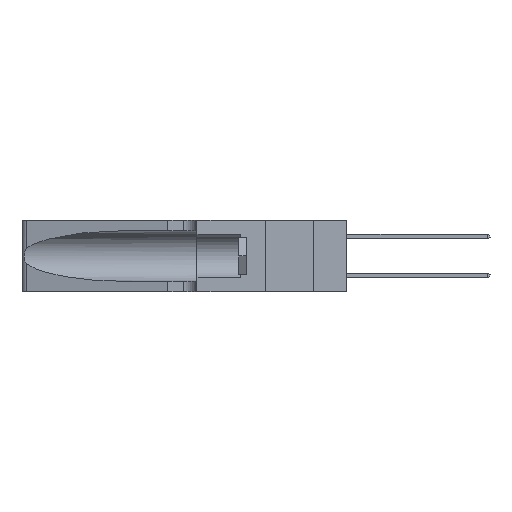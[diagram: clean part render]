
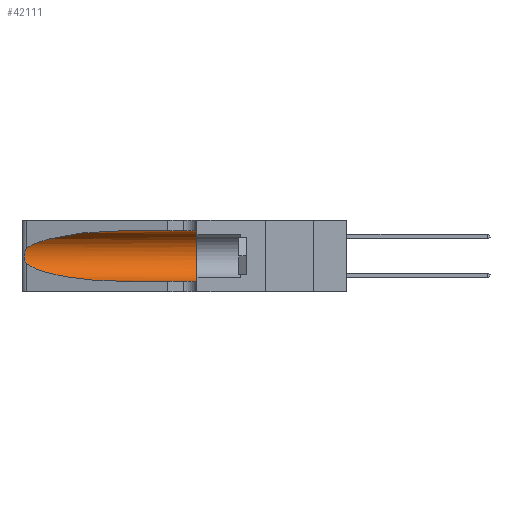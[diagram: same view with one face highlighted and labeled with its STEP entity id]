
A CAD part, left-side view. The second image highlights one B-rep face of the part: STEP entity #42111.
In plain terms, the highlighted cylindrical face has radius 3.308 mm (diameter 6.617 mm), a partial arc.
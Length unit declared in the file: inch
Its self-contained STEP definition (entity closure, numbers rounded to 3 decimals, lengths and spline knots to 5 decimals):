
#189 = DIRECTION ( 'NONE',  ( 0., -1., 0. ) ) ;
#308 = LINE ( 'NONE', #18726, #39827 ) ;
#416 = EDGE_CURVE ( 'NONE', #18022, #40459, #35039, .T. ) ;
#1142 = FACE_OUTER_BOUND ( 'NONE', #48727, .T. ) ;
#2144 = LINE ( 'NONE', #30897, #41596 ) ;
#3174 = CARTESIAN_POINT ( 'NONE',  ( 0.26075, 1.23896, 0.19203 ) ) ;
#3382 = DIRECTION ( 'NONE',  ( 0., 0., 1. ) ) ;
#7046 = CARTESIAN_POINT ( 'NONE',  ( 0.26017, 1.23833, 0.17102 ) ) ;
#7068 = VERTEX_POINT ( 'NONE', #26553 ) ;
#7631 = EDGE_CURVE ( 'NONE', #7068, #35175, #38457, .T. ) ;
#7908 = EDGE_CURVE ( 'NONE', #14435, #7068, #29641, .T. ) ;
#8144 =( BOUNDED_CURVE ( )  B_SPLINE_CURVE ( 3, ( #31786, #16528, #46935, #24254 ),
 .UNSPECIFIED., .F., .F. ) 
 B_SPLINE_CURVE_WITH_KNOTS ( ( 4, 4 ),
 ( 3.44316, 4.71239 ),
 .UNSPECIFIED. ) 
 CURVE ( )  GEOMETRIC_REPRESENTATION_ITEM ( )  RATIONAL_B_SPLINE_CURVE ( ( 1., 0.87, 0.87, 1. ) ) 
 REPRESENTATION_ITEM ( '' )  );
#10740 = CARTESIAN_POINT ( 'NONE',  ( 0.25555, 1.22994, 0.2215 ) ) ;
#10910 = CARTESIAN_POINT ( 'NONE',  ( 0.25789, 1.23486, 0.15765 ) ) ;
#12070 = ORIENTED_EDGE ( 'NONE', *, *, #41058, .T. ) ;
#12370 = CARTESIAN_POINT ( 'NONE',  ( 0.2373, 1.15595, 0.28018 ) ) ;
#14435 = VERTEX_POINT ( 'NONE', #36210 ) ;
#14732 = CARTESIAN_POINT ( 'NONE',  ( 0.25555, 1.22993, 0.14849 ) ) ;
#15264 = ORIENTED_EDGE ( 'NONE', *, *, #7908, .T. ) ;
#16361 = AXIS2_PLACEMENT_3D ( 'NONE', #46184, #19645, #23495 ) ;
#16528 = CARTESIAN_POINT ( 'NONE',  ( 0.2373, 1.15595, 0.08982 ) ) ;
#16903 = ORIENTED_EDGE ( 'NONE', *, *, #416, .F. ) ;
#17095 = ORIENTED_EDGE ( 'NONE', *, *, #7631, .T. ) ;
#18022 = VERTEX_POINT ( 'NONE', #38744 ) ;
#18726 = CARTESIAN_POINT ( 'NONE',  ( 0.1305, 1.61858, 0.31525 ) ) ;
#19645 = DIRECTION ( 'NONE',  ( 0., -1., 0. ) ) ;
#21640 = CARTESIAN_POINT ( 'NONE',  ( 0.25487, 1.22718, 0.14631 ) ) ;
#22294 = CARTESIAN_POINT ( 'NONE',  ( 0.25787, 1.23484, 0.2124 ) ) ;
#23495 = DIRECTION ( 'NONE',  ( 0., 0., -1. ) ) ;
#24254 = CARTESIAN_POINT ( 'NONE',  ( 0.1305, 0.72297, 0.05475 ) ) ;
#25541 = VERTEX_POINT ( 'NONE', #34522 ) ;
#26155 = CARTESIAN_POINT ( 'NONE',  ( 0.26018, 1.23835, 0.19895 ) ) ;
#26376 = DIRECTION ( 'NONE',  ( 0., 1., 0. ) ) ;
#26553 = CARTESIAN_POINT ( 'NONE',  ( 0.25487, 1.22718, 0.22369 ) ) ;
#27500 = EDGE_CURVE ( 'NONE', #25541, #40459, #2144, .T. ) ;
#29641 =( BOUNDED_CURVE ( )  B_SPLINE_CURVE ( 3, ( #31464, #35264, #12370, #39073 ),
 .UNSPECIFIED., .F., .T. ) 
 B_SPLINE_CURVE_WITH_KNOTS ( ( 4, 4 ),
 ( 1.5708, 2.84003 ),
 .UNSPECIFIED. ) 
 CURVE ( )  GEOMETRIC_REPRESENTATION_ITEM ( )  RATIONAL_B_SPLINE_CURVE ( ( 1., 0.87, 0.87, 1. ) ) 
 REPRESENTATION_ITEM ( '' )  );
#29834 = CARTESIAN_POINT ( 'NONE',  ( 0.25487, 1.22718, 0.22369 ) ) ;
#29999 = CARTESIAN_POINT ( 'NONE',  ( 0.26075, 1.23896, 0.178 ) ) ;
#30541 = CYLINDRICAL_SURFACE ( 'NONE', #16361, 0.13025 ) ;
#30897 = CARTESIAN_POINT ( 'NONE',  ( 0.1305, 1.61858, 0.05475 ) ) ;
#31464 = CARTESIAN_POINT ( 'NONE',  ( 0.1305, 0.72297, 0.31525 ) ) ;
#31786 = CARTESIAN_POINT ( 'NONE',  ( 0.25487, 1.22718, 0.14631 ) ) ;
#33821 = CARTESIAN_POINT ( 'NONE',  ( 0.25856, 1.23593, 0.16098 ) ) ;
#34254 = DIRECTION ( 'NONE',  ( 0., -1., 0. ) ) ;
#34522 = CARTESIAN_POINT ( 'NONE',  ( 0.1305, 0.72297, 0.05475 ) ) ;
#34576 = AXIS2_PLACEMENT_3D ( 'NONE', #49012, #26376, #3382 ) ;
#35039 = CIRCLE ( 'NONE', #34576, 0.13025 ) ;
#35175 = VERTEX_POINT ( 'NONE', #21640 ) ;
#35264 = CARTESIAN_POINT ( 'NONE',  ( 0.18966, 0.96281, 0.31525 ) ) ;
#36022 = ORIENTED_EDGE ( 'NONE', *, *, #27500, .T. ) ;
#36210 = CARTESIAN_POINT ( 'NONE',  ( 0.1305, 0.72297, 0.31525 ) ) ;
#37619 = CARTESIAN_POINT ( 'NONE',  ( 0.25639, 1.23186, 0.15144 ) ) ;
#38457 = B_SPLINE_CURVE_WITH_KNOTS ( 'NONE', 3,
 ( #29834, #10740, #45012, #22294, #48805, #26155, #3174, #29999, #7046, #33821, #10910, #37619, #14732, #41413 ),
 .UNSPECIFIED., .F., .F.,
 ( 4, 2, 2, 2, 2, 2, 4 ),
 ( 0., 0.00027, 0.00053, 0.00107, 0.0016, 0.00187, 0.00214 ),
 .UNSPECIFIED. ) ;
#38744 = CARTESIAN_POINT ( 'NONE',  ( 0.1305, 0.35, 0.31525 ) ) ;
#39073 = CARTESIAN_POINT ( 'NONE',  ( 0.25487, 1.22718, 0.22369 ) ) ;
#39827 = VECTOR ( 'NONE', #34254, 39.37008 ) ;
#40459 = VERTEX_POINT ( 'NONE', #43600 ) ;
#41058 = EDGE_CURVE ( 'NONE', #35175, #25541, #8144, .T. ) ;
#41413 = CARTESIAN_POINT ( 'NONE',  ( 0.25487, 1.22718, 0.14631 ) ) ;
#41596 = VECTOR ( 'NONE', #189, 39.37008 ) ;
#42111 = ADVANCED_FACE ( 'NONE', ( #1142 ), #30541, .F. ) ;
#43600 = CARTESIAN_POINT ( 'NONE',  ( 0.1305, 0.35, 0.05475 ) ) ;
#44802 = EDGE_CURVE ( 'NONE', #14435, #18022, #308, .T. ) ;
#45012 = CARTESIAN_POINT ( 'NONE',  ( 0.25639, 1.23184, 0.21858 ) ) ;
#45108 = ORIENTED_EDGE ( 'NONE', *, *, #44802, .F. ) ;
#46184 = CARTESIAN_POINT ( 'NONE',  ( 0.1305, 1.61858, 0.185 ) ) ;
#46935 = CARTESIAN_POINT ( 'NONE',  ( 0.18966, 0.96281, 0.05475 ) ) ;
#48727 = EDGE_LOOP ( 'NONE', ( #15264, #17095, #12070, #36022, #16903, #45108 ) ) ;
#48805 = CARTESIAN_POINT ( 'NONE',  ( 0.25854, 1.2359, 0.20912 ) ) ;
#49012 = CARTESIAN_POINT ( 'NONE',  ( 0.1305, 0.35, 0.185 ) ) ;
